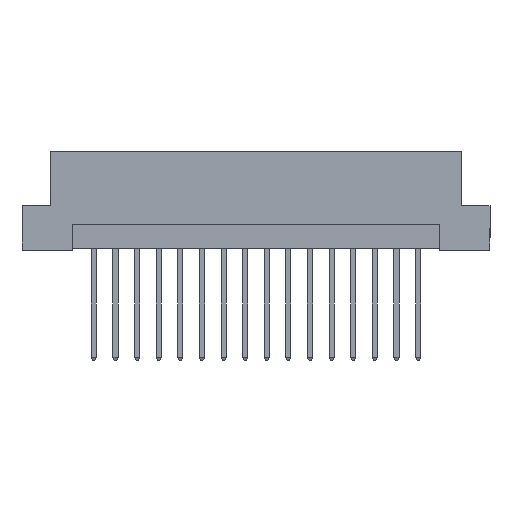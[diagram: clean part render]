
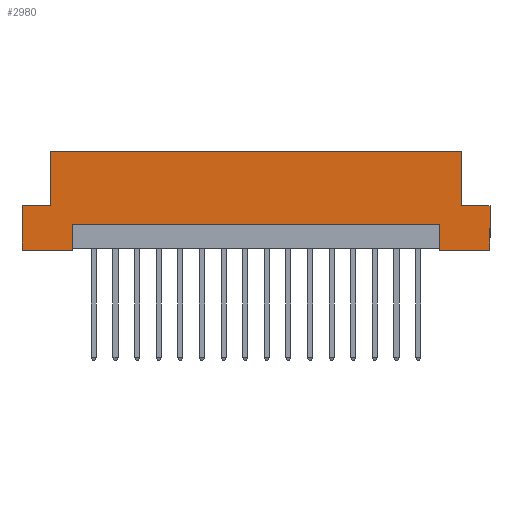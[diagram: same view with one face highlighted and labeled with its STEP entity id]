
A CAD part, front view. The second image highlights one B-rep face of the part: STEP entity #2980.
In plain terms, the highlighted planar face has unit normal (0, -1, 0).
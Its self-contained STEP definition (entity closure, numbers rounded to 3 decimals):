
#12 = PLANE ( 'NONE',  #386 ) ;
#25 = CARTESIAN_POINT ( 'NONE',  ( -21.6, -4.3, 0.2 ) ) ;
#100 = VECTOR ( 'NONE', #6009, 1000. ) ;
#150 = CARTESIAN_POINT ( 'NONE',  ( -21.6, -4.3, 3. ) ) ;
#222 = VECTOR ( 'NONE', #632, 1000. ) ;
#243 = CARTESIAN_POINT ( 'NONE',  ( 27.5, -4.3, 0. ) ) ;
#257 = DIRECTION ( 'NONE',  ( 1., 0., 0. ) ) ;
#386 = AXIS2_PLACEMENT_3D ( 'NONE', #4210, #2156, #4312 ) ;
#592 = LINE ( 'NONE', #3307, #5028 ) ;
#629 = DIRECTION ( 'NONE',  ( 0., 0., -1. ) ) ;
#632 = DIRECTION ( 'NONE',  ( 0., 0., -1. ) ) ;
#645 = CARTESIAN_POINT ( 'NONE',  ( 21.6, -4.3, 0.2 ) ) ;
#764 = VERTEX_POINT ( 'NONE', #4331 ) ;
#870 = ORIENTED_EDGE ( 'NONE', *, *, #2167, .F. ) ;
#979 = CARTESIAN_POINT ( 'NONE',  ( -24.2, -4.3, 5.2 ) ) ;
#1121 = VECTOR ( 'NONE', #2830, 1000. ) ;
#1137 = EDGE_CURVE ( 'NONE', #5126, #3107, #592, .T. ) ;
#1164 = DIRECTION ( 'NONE',  ( 1., 0., 0. ) ) ;
#1225 = EDGE_CURVE ( 'NONE', #6894, #6140, #2170, .T. ) ;
#1298 = ORIENTED_EDGE ( 'NONE', *, *, #2543, .T. ) ;
#1340 = CARTESIAN_POINT ( 'NONE',  ( 24.2, -4.3, 5.2 ) ) ;
#1485 = LINE ( 'NONE', #4319, #6390 ) ;
#1535 = EDGE_CURVE ( 'NONE', #4425, #6930, #5083, .T. ) ;
#1574 = LINE ( 'NONE', #4840, #4984 ) ;
#1597 = ORIENTED_EDGE ( 'NONE', *, *, #5880, .F. ) ;
#1765 = EDGE_CURVE ( 'NONE', #5126, #5897, #2294, .T. ) ;
#1847 = CARTESIAN_POINT ( 'NONE',  ( 27.5, -4.3, 11.6 ) ) ;
#1973 = ORIENTED_EDGE ( 'NONE', *, *, #6749, .T. ) ;
#2156 = DIRECTION ( 'NONE',  ( 0., 1., 0. ) ) ;
#2167 = EDGE_CURVE ( 'NONE', #2639, #4425, #6307, .T. ) ;
#2170 = LINE ( 'NONE', #25, #6490 ) ;
#2217 = LINE ( 'NONE', #2791, #1121 ) ;
#2294 = LINE ( 'NONE', #645, #5761 ) ;
#2333 = EDGE_LOOP ( 'NONE', ( #1298, #4449, #6673, #3066, #6646, #5311, #5925, #870, #1597, #1973, #3294, #6591 ) ) ;
#2543 = EDGE_CURVE ( 'NONE', #6894, #5897, #1485, .T. ) ;
#2639 = VERTEX_POINT ( 'NONE', #979 ) ;
#2791 = CARTESIAN_POINT ( 'NONE',  ( 27.5, -4.3, 5.2 ) ) ;
#2830 = DIRECTION ( 'NONE',  ( 1., 0., 0. ) ) ;
#2912 = VECTOR ( 'NONE', #3703, 1000. ) ;
#2980 = ADVANCED_FACE ( 'NONE', ( #4841 ), #12, .F. ) ;
#3066 = ORIENTED_EDGE ( 'NONE', *, *, #4107, .F. ) ;
#3096 = VECTOR ( 'NONE', #6718, 1000. ) ;
#3107 = VERTEX_POINT ( 'NONE', #3362 ) ;
#3231 = LINE ( 'NONE', #3795, #100 ) ;
#3274 = LINE ( 'NONE', #5410, #222 ) ;
#3294 = ORIENTED_EDGE ( 'NONE', *, *, #3689, .T. ) ;
#3307 = CARTESIAN_POINT ( 'NONE',  ( 27.5, -4.3, 0. ) ) ;
#3362 = CARTESIAN_POINT ( 'NONE',  ( 27.5, -4.3, 0. ) ) ;
#3550 = VERTEX_POINT ( 'NONE', #4972 ) ;
#3669 = CARTESIAN_POINT ( 'NONE',  ( -27.5, -4.3, 0. ) ) ;
#3689 = EDGE_CURVE ( 'NONE', #4660, #6140, #4547, .T. ) ;
#3703 = DIRECTION ( 'NONE',  ( 0., 0., 1. ) ) ;
#3795 = CARTESIAN_POINT ( 'NONE',  ( -27.5, -4.3, 5.2 ) ) ;
#3865 = CARTESIAN_POINT ( 'NONE',  ( -24.2, -4.3, 11.6 ) ) ;
#4107 = EDGE_CURVE ( 'NONE', #3550, #3107, #3274, .T. ) ;
#4210 = CARTESIAN_POINT ( 'NONE',  ( 27.5, -4.3, 11.6 ) ) ;
#4312 = DIRECTION ( 'NONE',  ( -1., 0., 0. ) ) ;
#4319 = CARTESIAN_POINT ( 'NONE',  ( -21.6, -4.3, 3. ) ) ;
#4331 = CARTESIAN_POINT ( 'NONE',  ( 24.2, -4.3, 5.2 ) ) ;
#4425 = VERTEX_POINT ( 'NONE', #3865 ) ;
#4445 = DIRECTION ( 'NONE',  ( 0., 0., 1. ) ) ;
#4449 = ORIENTED_EDGE ( 'NONE', *, *, #1765, .F. ) ;
#4482 = CARTESIAN_POINT ( 'NONE',  ( 24.2, -4.3, 11.6 ) ) ;
#4547 = LINE ( 'NONE', #243, #3096 ) ;
#4638 = CARTESIAN_POINT ( 'NONE',  ( -21.6, -4.3, 0. ) ) ;
#4660 = VERTEX_POINT ( 'NONE', #3669 ) ;
#4829 = EDGE_CURVE ( 'NONE', #764, #3550, #2217, .T. ) ;
#4840 = CARTESIAN_POINT ( 'NONE',  ( -27.5, -4.3, 11.6 ) ) ;
#4841 = FACE_OUTER_BOUND ( 'NONE', #2333, .T. ) ;
#4856 = CARTESIAN_POINT ( 'NONE',  ( 21.6, -4.3, 3. ) ) ;
#4972 = CARTESIAN_POINT ( 'NONE',  ( 27.5, -4.3, 5.2 ) ) ;
#4984 = VECTOR ( 'NONE', #6482, 1000. ) ;
#5028 = VECTOR ( 'NONE', #1164, 1000. ) ;
#5083 = LINE ( 'NONE', #1847, #6293 ) ;
#5124 = DIRECTION ( 'NONE',  ( 0., 0., 1. ) ) ;
#5126 = VERTEX_POINT ( 'NONE', #5736 ) ;
#5267 = DIRECTION ( 'NONE',  ( 1., 0., 0. ) ) ;
#5311 = ORIENTED_EDGE ( 'NONE', *, *, #5494, .T. ) ;
#5410 = CARTESIAN_POINT ( 'NONE',  ( 27.5, -4.3, 11.6 ) ) ;
#5494 = EDGE_CURVE ( 'NONE', #764, #6930, #6676, .T. ) ;
#5499 = VERTEX_POINT ( 'NONE', #5622 ) ;
#5622 = CARTESIAN_POINT ( 'NONE',  ( -27.5, -4.3, 5.2 ) ) ;
#5736 = CARTESIAN_POINT ( 'NONE',  ( 21.6, -4.3, 0. ) ) ;
#5761 = VECTOR ( 'NONE', #4445, 1000. ) ;
#5880 = EDGE_CURVE ( 'NONE', #5499, #2639, #3231, .T. ) ;
#5897 = VERTEX_POINT ( 'NONE', #4856 ) ;
#5925 = ORIENTED_EDGE ( 'NONE', *, *, #1535, .F. ) ;
#6009 = DIRECTION ( 'NONE',  ( 1., 0., 0. ) ) ;
#6140 = VERTEX_POINT ( 'NONE', #4638 ) ;
#6293 = VECTOR ( 'NONE', #257, 1000. ) ;
#6307 = LINE ( 'NONE', #6370, #2912 ) ;
#6370 = CARTESIAN_POINT ( 'NONE',  ( -24.2, -4.3, 5.2 ) ) ;
#6390 = VECTOR ( 'NONE', #5267, 1000. ) ;
#6396 = VECTOR ( 'NONE', #5124, 1000. ) ;
#6482 = DIRECTION ( 'NONE',  ( 0., 0., -1. ) ) ;
#6490 = VECTOR ( 'NONE', #629, 1000. ) ;
#6591 = ORIENTED_EDGE ( 'NONE', *, *, #1225, .F. ) ;
#6646 = ORIENTED_EDGE ( 'NONE', *, *, #4829, .F. ) ;
#6673 = ORIENTED_EDGE ( 'NONE', *, *, #1137, .T. ) ;
#6676 = LINE ( 'NONE', #1340, #6396 ) ;
#6718 = DIRECTION ( 'NONE',  ( 1., 0., 0. ) ) ;
#6749 = EDGE_CURVE ( 'NONE', #5499, #4660, #1574, .T. ) ;
#6894 = VERTEX_POINT ( 'NONE', #150 ) ;
#6930 = VERTEX_POINT ( 'NONE', #4482 ) ;
